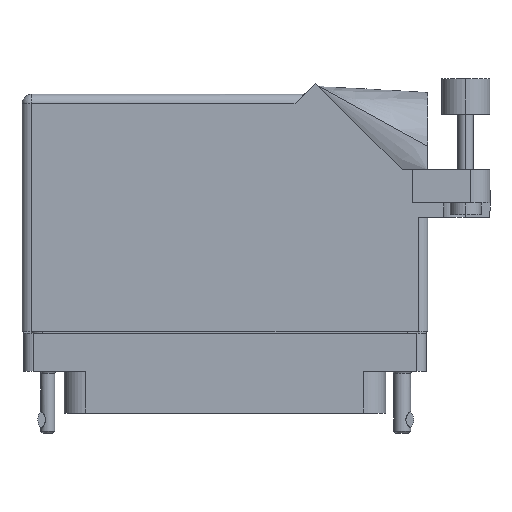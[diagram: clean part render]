
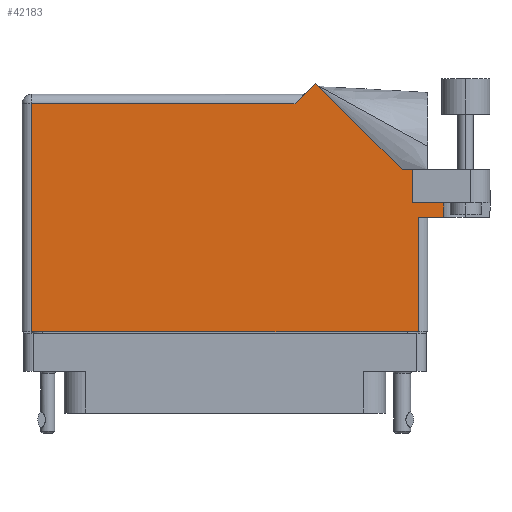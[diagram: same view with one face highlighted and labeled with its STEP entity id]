
A CAD part, front view. The second image highlights one B-rep face of the part: STEP entity #42183.
In plain terms, the highlighted face is planar.
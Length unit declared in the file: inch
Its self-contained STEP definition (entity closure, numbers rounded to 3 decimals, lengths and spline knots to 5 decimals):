
#1208 = VERTEX_POINT ( 'NONE', #23630 ) ;
#1457 = EDGE_CURVE ( 'NONE', #11492, #28569, #39524, .T. ) ;
#1736 = EDGE_LOOP ( 'NONE', ( #15952, #52274, #15070, #19640, #18894, #18258, #33773, #50716, #42551, #15133, #11178 ) ) ;
#3271 = DIRECTION ( 'NONE',  ( 0., 1., 0. ) ) ;
#4308 = VECTOR ( 'NONE', #53576, 39.37008 ) ;
#6361 = VERTEX_POINT ( 'NONE', #11633 ) ;
#6638 = VECTOR ( 'NONE', #60564, 39.37008 ) ;
#6859 = DIRECTION ( 'NONE',  ( -1., 0., 0. ) ) ;
#7582 = LINE ( 'NONE', #39651, #46980 ) ;
#8187 = CARTESIAN_POINT ( 'NONE',  ( 1.14042, 0.944, 0.455 ) ) ;
#9500 = PLANE ( 'NONE',  #13859 ) ;
#9939 = VERTEX_POINT ( 'NONE', #41122 ) ;
#9966 = LINE ( 'NONE', #37618, #52979 ) ;
#10542 = CARTESIAN_POINT ( 'NONE',  ( 1.244, 0.637, 0.455 ) ) ;
#11178 = ORIENTED_EDGE ( 'NONE', *, *, #55809, .T. ) ;
#11492 = VERTEX_POINT ( 'NONE', #37551 ) ;
#11633 = CARTESIAN_POINT ( 'NONE',  ( -1.244, 1.368, 0.455 ) ) ;
#12138 = VECTOR ( 'NONE', #55667, 39.37008 ) ;
#13138 = DIRECTION ( 'NONE',  ( 0., -1., 0. ) ) ;
#13408 = CARTESIAN_POINT ( 'NONE',  ( 1.4075, 0.637, 0.455 ) ) ;
#13859 = AXIS2_PLACEMENT_3D ( 'NONE', #19733, #48111, #24672 ) ;
#15070 = ORIENTED_EDGE ( 'NONE', *, *, #60415, .T. ) ;
#15133 = ORIENTED_EDGE ( 'NONE', *, *, #57897, .T. ) ;
#15952 = ORIENTED_EDGE ( 'NONE', *, *, #24910, .T. ) ;
#17435 = CARTESIAN_POINT ( 'NONE',  ( 1.244, 0.637, 0.455 ) ) ;
#18258 = ORIENTED_EDGE ( 'NONE', *, *, #51075, .T. ) ;
#18396 = CARTESIAN_POINT ( 'NONE',  ( 0.58371, 1.50071, 0.455 ) ) ;
#18894 = ORIENTED_EDGE ( 'NONE', *, *, #33867, .F. ) ;
#19323 = LINE ( 'NONE', #22684, #6638 ) ;
#19640 = ORIENTED_EDGE ( 'NONE', *, *, #20747, .F. ) ;
#19733 = CARTESIAN_POINT ( 'NONE',  ( -1.306, 1.43, 0.455 ) ) ;
#20747 = EDGE_CURVE ( 'NONE', #41026, #47334, #34014, .T. ) ;
#21299 = CARTESIAN_POINT ( 'NONE',  ( 1.244, -0.1, 0.455 ) ) ;
#21849 = FACE_OUTER_BOUND ( 'NONE', #1736, .T. ) ;
#22684 = CARTESIAN_POINT ( 'NONE',  ( 1.306, 0.637, 0.455 ) ) ;
#23630 = CARTESIAN_POINT ( 'NONE',  ( 1.206, 0.944, 0.455 ) ) ;
#24006 = LINE ( 'NONE', #41004, #12138 ) ;
#24014 = CARTESIAN_POINT ( 'NONE',  ( 0.513, 1.43, 0.455 ) ) ;
#24672 = DIRECTION ( 'NONE',  ( -1., 0., 0. ) ) ;
#24695 = EDGE_CURVE ( 'NONE', #55642, #34548, #27014, .T. ) ;
#24910 = EDGE_CURVE ( 'NONE', #9939, #55642, #24006, .T. ) ;
#25198 = CARTESIAN_POINT ( 'NONE',  ( 1.206, 0.731, 0.455 ) ) ;
#25449 = DIRECTION ( 'NONE',  ( 1., 0., 0. ) ) ;
#26094 = LINE ( 'NONE', #25198, #39442 ) ;
#26839 = CARTESIAN_POINT ( 'NONE',  ( 1.4075, 1.06177, 0.455 ) ) ;
#27014 = LINE ( 'NONE', #17435, #27699 ) ;
#27699 = VECTOR ( 'NONE', #3271, 39.37008 ) ;
#28569 = VERTEX_POINT ( 'NONE', #18396 ) ;
#33569 = CARTESIAN_POINT ( 'NONE',  ( 1.706, 0.944, 0.455 ) ) ;
#33773 = ORIENTED_EDGE ( 'NONE', *, *, #59019, .T. ) ;
#33867 = EDGE_CURVE ( 'NONE', #60006, #41026, #54135, .T. ) ;
#34014 = LINE ( 'NONE', #26839, #48916 ) ;
#34548 = VERTEX_POINT ( 'NONE', #10542 ) ;
#35114 = EDGE_CURVE ( 'NONE', #28569, #56509, #41427, .T. ) ;
#35988 = DIRECTION ( 'NONE',  ( -0.707, 0.707, 0. ) ) ;
#36983 = DIRECTION ( 'NONE',  ( 0., -1., 0. ) ) ;
#37551 = CARTESIAN_POINT ( 'NONE',  ( 1.14042, 0.944, 0.455 ) ) ;
#37618 = CARTESIAN_POINT ( 'NONE',  ( -1.244, -0.1, 0.455 ) ) ;
#38560 = DIRECTION ( 'NONE',  ( -1., 0., 0. ) ) ;
#39442 = VECTOR ( 'NONE', #48443, 39.37008 ) ;
#39524 = LINE ( 'NONE', #8187, #56567 ) ;
#39651 = CARTESIAN_POINT ( 'NONE',  ( -1.306, 1.368, 0.455 ) ) ;
#40157 = VECTOR ( 'NONE', #38560, 39.37008 ) ;
#40613 = CARTESIAN_POINT ( 'NONE',  ( 1.206, 0.731, 0.455 ) ) ;
#41004 = CARTESIAN_POINT ( 'NONE',  ( -1.306, -0.1, 0.455 ) ) ;
#41026 = VERTEX_POINT ( 'NONE', #43840 ) ;
#41122 = CARTESIAN_POINT ( 'NONE',  ( -1.244, -0.1, 0.455 ) ) ;
#41427 = LINE ( 'NONE', #24014, #4308 ) ;
#42183 = ADVANCED_FACE ( 'NONE', ( #21849 ), #9500, .F. ) ;
#42551 = ORIENTED_EDGE ( 'NONE', *, *, #35114, .T. ) ;
#43780 = VECTOR ( 'NONE', #25449, 39.37008 ) ;
#43840 = CARTESIAN_POINT ( 'NONE',  ( 1.4075, 0.731, 0.455 ) ) ;
#44718 = CARTESIAN_POINT ( 'NONE',  ( 1.206, 0.731, 0.455 ) ) ;
#46545 = CARTESIAN_POINT ( 'NONE',  ( 0.451, 1.368, 0.455 ) ) ;
#46980 = VECTOR ( 'NONE', #6859, 39.37008 ) ;
#47334 = VERTEX_POINT ( 'NONE', #13408 ) ;
#48111 = DIRECTION ( 'NONE',  ( 0., 0., -1. ) ) ;
#48443 = DIRECTION ( 'NONE',  ( 0., 1., 0. ) ) ;
#48916 = VECTOR ( 'NONE', #36983, 39.37008 ) ;
#50716 = ORIENTED_EDGE ( 'NONE', *, *, #1457, .T. ) ;
#51075 = EDGE_CURVE ( 'NONE', #60006, #1208, #26094, .T. ) ;
#52274 = ORIENTED_EDGE ( 'NONE', *, *, #24695, .T. ) ;
#52737 = LINE ( 'NONE', #33569, #40157 ) ;
#52979 = VECTOR ( 'NONE', #13138, 39.37008 ) ;
#53576 = DIRECTION ( 'NONE',  ( -0.707, -0.707, 0. ) ) ;
#54135 = LINE ( 'NONE', #44718, #43780 ) ;
#55642 = VERTEX_POINT ( 'NONE', #21299 ) ;
#55667 = DIRECTION ( 'NONE',  ( 1., 0., 0. ) ) ;
#55809 = EDGE_CURVE ( 'NONE', #6361, #9939, #9966, .T. ) ;
#56509 = VERTEX_POINT ( 'NONE', #46545 ) ;
#56567 = VECTOR ( 'NONE', #35988, 39.37008 ) ;
#57897 = EDGE_CURVE ( 'NONE', #56509, #6361, #7582, .T. ) ;
#59019 = EDGE_CURVE ( 'NONE', #1208, #11492, #52737, .T. ) ;
#60006 = VERTEX_POINT ( 'NONE', #40613 ) ;
#60415 = EDGE_CURVE ( 'NONE', #34548, #47334, #19323, .T. ) ;
#60564 = DIRECTION ( 'NONE',  ( 1., 0., 0. ) ) ;
